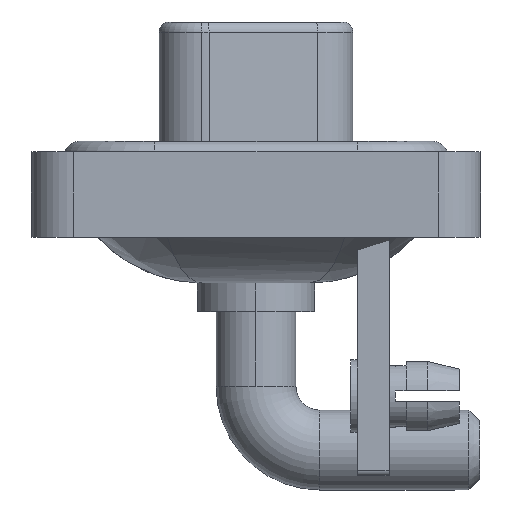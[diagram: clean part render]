
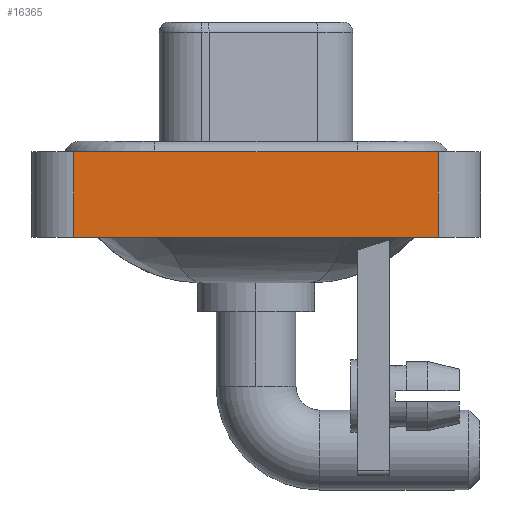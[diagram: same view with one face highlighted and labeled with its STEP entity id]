
A CAD part, left-side view. The second image highlights one B-rep face of the part: STEP entity #16365.
In plain terms, the highlighted planar face has unit normal (-1, 0, 0).
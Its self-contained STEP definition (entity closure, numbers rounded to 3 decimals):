
#334 = ORIENTED_EDGE ( 'NONE', *, *, #17719, .F. ) ;
#1292 = CARTESIAN_POINT ( 'NONE',  ( -7.25, 8.55, 0.4 ) ) ;
#1307 = ORIENTED_EDGE ( 'NONE', *, *, #2896, .T. ) ;
#1356 = ORIENTED_EDGE ( 'NONE', *, *, #6995, .T. ) ;
#1358 = VECTOR ( 'NONE', #13157, 1000. ) ;
#2288 = VERTEX_POINT ( 'NONE', #4507 ) ;
#2296 = LINE ( 'NONE', #11750, #9814 ) ;
#2896 = EDGE_CURVE ( 'NONE', #2288, #19704, #2296, .T. ) ;
#3228 = AXIS2_PLACEMENT_3D ( 'NONE', #18146, #13341, #4204 ) ;
#3655 = VECTOR ( 'NONE', #13446, 1000. ) ;
#4204 = DIRECTION ( 'NONE',  ( 0., 0., 1. ) ) ;
#4507 = CARTESIAN_POINT ( 'NONE',  ( -7.25, 8.55, -3.6 ) ) ;
#4559 = VERTEX_POINT ( 'NONE', #16772 ) ;
#5455 = VERTEX_POINT ( 'NONE', #1292 ) ;
#5498 = CARTESIAN_POINT ( 'NONE',  ( -7.25, -8.55, -3.6 ) ) ;
#5755 = LINE ( 'NONE', #16443, #3655 ) ;
#6995 = EDGE_CURVE ( 'NONE', #19704, #4559, #15222, .T. ) ;
#8425 = LINE ( 'NONE', #9868, #1358 ) ;
#8696 = CARTESIAN_POINT ( 'NONE',  ( -7.25, -8.55, -3.6 ) ) ;
#9814 = VECTOR ( 'NONE', #13182, 1000. ) ;
#9868 = CARTESIAN_POINT ( 'NONE',  ( -7.25, 8.55, -3.6 ) ) ;
#11750 = CARTESIAN_POINT ( 'NONE',  ( -7.25, -8.55, -3.6 ) ) ;
#11875 = DIRECTION ( 'NONE',  ( 0., 0., 1. ) ) ;
#12876 = EDGE_LOOP ( 'NONE', ( #1356, #334, #19057, #1307 ) ) ;
#13157 = DIRECTION ( 'NONE',  ( 0., 0., 1. ) ) ;
#13182 = DIRECTION ( 'NONE',  ( 0., -1., 0. ) ) ;
#13247 = FACE_OUTER_BOUND ( 'NONE', #12876, .T. ) ;
#13341 = DIRECTION ( 'NONE',  ( -1., 0., 0. ) ) ;
#13443 = PLANE ( 'NONE',  #3228 ) ;
#13446 = DIRECTION ( 'NONE',  ( 0., -1., 0. ) ) ;
#15222 = LINE ( 'NONE', #5498, #16659 ) ;
#16365 = ADVANCED_FACE ( 'NONE', ( #13247 ), #13443, .T. ) ;
#16443 = CARTESIAN_POINT ( 'NONE',  ( -7.25, -8.55, 0.4 ) ) ;
#16659 = VECTOR ( 'NONE', #11875, 1000. ) ;
#16772 = CARTESIAN_POINT ( 'NONE',  ( -7.25, -8.55, 0.4 ) ) ;
#17585 = EDGE_CURVE ( 'NONE', #2288, #5455, #8425, .T. ) ;
#17719 = EDGE_CURVE ( 'NONE', #5455, #4559, #5755, .T. ) ;
#18146 = CARTESIAN_POINT ( 'NONE',  ( -7.25, -8.55, -3.6 ) ) ;
#19057 = ORIENTED_EDGE ( 'NONE', *, *, #17585, .F. ) ;
#19704 = VERTEX_POINT ( 'NONE', #8696 ) ;
